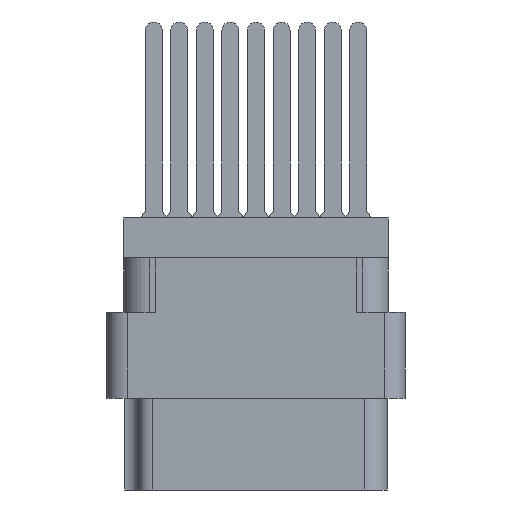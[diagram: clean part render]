
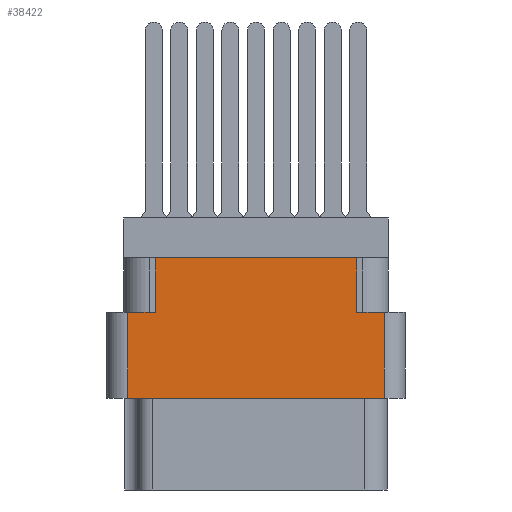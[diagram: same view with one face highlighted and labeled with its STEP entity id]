
A CAD part, left-side view. The second image highlights one B-rep face of the part: STEP entity #38422.
In plain terms, the highlighted planar face has unit normal (-1, 0, 0).
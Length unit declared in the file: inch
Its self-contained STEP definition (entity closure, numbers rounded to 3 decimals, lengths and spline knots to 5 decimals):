
#3 = CARTESIAN_POINT ( 'NONE',  ( -1.296, -0.376, -0.277 ) ) ;
#1250 = LINE ( 'NONE', #6224, #28453 ) ;
#2073 = VERTEX_POINT ( 'NONE', #26163 ) ;
#2764 = LINE ( 'NONE', #32431, #49123 ) ;
#4215 = FACE_OUTER_BOUND ( 'NONE', #28851, .T. ) ;
#5362 = ORIENTED_EDGE ( 'NONE', *, *, #36260, .F. ) ;
#5724 = VERTEX_POINT ( 'NONE', #33386 ) ;
#6224 = CARTESIAN_POINT ( 'NONE',  ( -1.296, 0., -0.277 ) ) ;
#6729 = CARTESIAN_POINT ( 'NONE',  ( -1.296, -0.376, -0.529 ) ) ;
#8041 = CARTESIAN_POINT ( 'NONE',  ( -1.296, 0., -0.277 ) ) ;
#8104 = CARTESIAN_POINT ( 'NONE',  ( -1.296, 0.438, -0.117 ) ) ;
#13271 = DIRECTION ( 'NONE',  ( 0., 0., -1. ) ) ;
#13532 = CARTESIAN_POINT ( 'NONE',  ( -1.296, -0.438, -0.798 ) ) ;
#13881 = VERTEX_POINT ( 'NONE', #19231 ) ;
#14513 = DIRECTION ( 'NONE',  ( 0., -1., 0. ) ) ;
#15594 = AXIS2_PLACEMENT_3D ( 'NONE', #13532, #48280, #24174 ) ;
#15743 = DIRECTION ( 'NONE',  ( 0., 0., 1. ) ) ;
#16420 = VERTEX_POINT ( 'NONE', #21198 ) ;
#17707 = EDGE_CURVE ( 'NONE', #34869, #2073, #2764, .T. ) ;
#17813 = ORIENTED_EDGE ( 'NONE', *, *, #23679, .F. ) ;
#18018 = VECTOR ( 'NONE', #35639, 39.37008 ) ;
#18085 = VECTOR ( 'NONE', #33952, 39.37008 ) ;
#18184 = CARTESIAN_POINT ( 'NONE',  ( -1.296, -0.376, -0.798 ) ) ;
#18900 = DIRECTION ( 'NONE',  ( 0., 1., 0. ) ) ;
#19231 = CARTESIAN_POINT ( 'NONE',  ( -1.296, 0.296, -0.117 ) ) ;
#20705 = VECTOR ( 'NONE', #15743, 39.37008 ) ;
#20987 = ORIENTED_EDGE ( 'NONE', *, *, #17707, .T. ) ;
#21198 = CARTESIAN_POINT ( 'NONE',  ( -1.296, -0.296, -0.117 ) ) ;
#21364 = CARTESIAN_POINT ( 'NONE',  ( -1.296, 0.376, -0.277 ) ) ;
#21556 = VERTEX_POINT ( 'NONE', #3 ) ;
#22166 = DIRECTION ( 'NONE',  ( 0., 0., 1. ) ) ;
#23679 = EDGE_CURVE ( 'NONE', #28367, #2073, #33210, .T. ) ;
#24174 = DIRECTION ( 'NONE',  ( 0., 0., 1. ) ) ;
#24670 = VERTEX_POINT ( 'NONE', #31575 ) ;
#25423 = ORIENTED_EDGE ( 'NONE', *, *, #30232, .T. ) ;
#26104 = VECTOR ( 'NONE', #22166, 39.37008 ) ;
#26163 = CARTESIAN_POINT ( 'NONE',  ( -1.296, 0.376, -0.529 ) ) ;
#28367 = VERTEX_POINT ( 'NONE', #6729 ) ;
#28453 = VECTOR ( 'NONE', #14513, 39.37008 ) ;
#28562 = PLANE ( 'NONE',  #15594 ) ;
#28851 = EDGE_LOOP ( 'NONE', ( #39717, #20987, #17813, #25423, #5362, #38289, #38088, #39406 ) ) ;
#30232 = EDGE_CURVE ( 'NONE', #28367, #21556, #43412, .T. ) ;
#30291 = VECTOR ( 'NONE', #43837, 39.37008 ) ;
#31575 = CARTESIAN_POINT ( 'NONE',  ( -1.296, 0.296, -0.277 ) ) ;
#32431 = CARTESIAN_POINT ( 'NONE',  ( -1.296, 0.376, -0.798 ) ) ;
#33210 = LINE ( 'NONE', #37554, #41231 ) ;
#33386 = CARTESIAN_POINT ( 'NONE',  ( -1.296, -0.296, -0.277 ) ) ;
#33952 = DIRECTION ( 'NONE',  ( 0., 0., 1. ) ) ;
#34869 = VERTEX_POINT ( 'NONE', #21364 ) ;
#34972 = EDGE_CURVE ( 'NONE', #5724, #16420, #49596, .T. ) ;
#35639 = DIRECTION ( 'NONE',  ( 0., -1., 0. ) ) ;
#36157 = LINE ( 'NONE', #39345, #20705 ) ;
#36260 = EDGE_CURVE ( 'NONE', #5724, #21556, #1250, .T. ) ;
#36556 = LINE ( 'NONE', #8041, #18018 ) ;
#37554 = CARTESIAN_POINT ( 'NONE',  ( -1.296, 0., -0.529 ) ) ;
#38088 = ORIENTED_EDGE ( 'NONE', *, *, #47266, .F. ) ;
#38289 = ORIENTED_EDGE ( 'NONE', *, *, #34972, .T. ) ;
#38396 = CARTESIAN_POINT ( 'NONE',  ( -1.296, -0.296, -0.277 ) ) ;
#38422 = ADVANCED_FACE ( 'NONE', ( #4215 ), #28562, .T. ) ;
#38943 = LINE ( 'NONE', #8104, #30291 ) ;
#39345 = CARTESIAN_POINT ( 'NONE',  ( -1.296, 0.296, -0.277 ) ) ;
#39406 = ORIENTED_EDGE ( 'NONE', *, *, #45814, .F. ) ;
#39717 = ORIENTED_EDGE ( 'NONE', *, *, #41338, .F. ) ;
#41231 = VECTOR ( 'NONE', #18900, 39.37008 ) ;
#41338 = EDGE_CURVE ( 'NONE', #34869, #24670, #36556, .T. ) ;
#43412 = LINE ( 'NONE', #18184, #26104 ) ;
#43837 = DIRECTION ( 'NONE',  ( 0., -1., 0. ) ) ;
#45814 = EDGE_CURVE ( 'NONE', #24670, #13881, #36157, .T. ) ;
#47266 = EDGE_CURVE ( 'NONE', #13881, #16420, #38943, .T. ) ;
#48280 = DIRECTION ( 'NONE',  ( -1., 0., 0. ) ) ;
#49123 = VECTOR ( 'NONE', #13271, 39.37008 ) ;
#49596 = LINE ( 'NONE', #38396, #18085 ) ;
